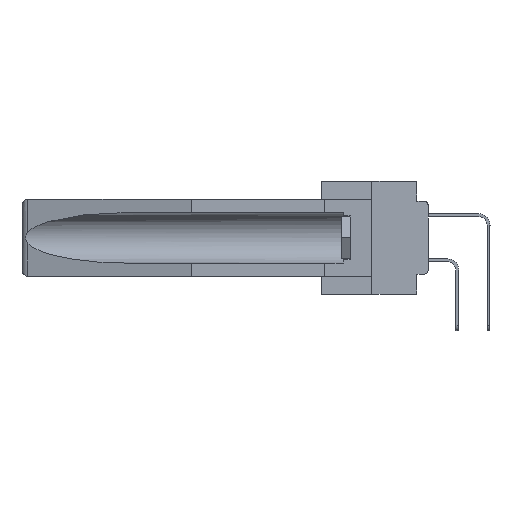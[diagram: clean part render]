
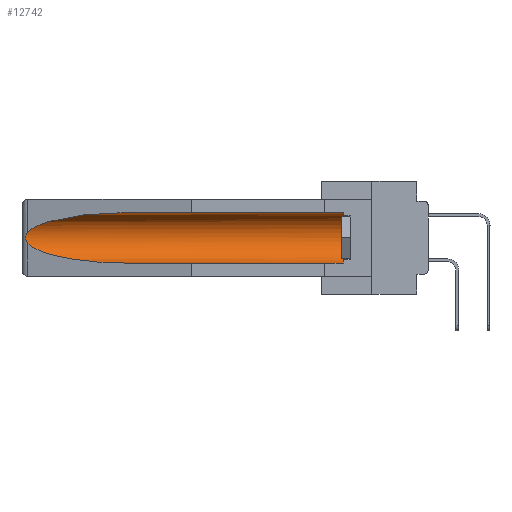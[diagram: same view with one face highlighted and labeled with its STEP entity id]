
A CAD part, left-side view. The second image highlights one B-rep face of the part: STEP entity #12742.
In plain terms, the highlighted cylindrical face has radius 2.857 mm (diameter 5.715 mm), a partial arc.
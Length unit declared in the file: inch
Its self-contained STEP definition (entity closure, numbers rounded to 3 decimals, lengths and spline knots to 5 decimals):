
#198 = CARTESIAN_POINT ( 'NONE',  ( 0.2675, 1.53308, -0.17534 ) ) ;
#292 = EDGE_CURVE ( 'NONE', #12893, #26331, #24643, .T. ) ;
#403 = CARTESIAN_POINT ( 'NONE',  ( 0.26537, 1.52718, -0.14972 ) ) ;
#547 = FACE_OUTER_BOUND ( 'NONE', #8751, .T. ) ;
#893 = CARTESIAN_POINT ( 'NONE',  ( 0.25451, 1.48313, -0.09465 ) ) ;
#2131 = CARTESIAN_POINT ( 'NONE',  ( 0.155, 0.126, -0.284 ) ) ;
#2896 = AXIS2_PLACEMENT_3D ( 'NONE', #5522, #5727, #15255 ) ;
#4227 = CARTESIAN_POINT ( 'NONE',  ( 0.155, 1.07973, -0.059 ) ) ;
#5254 = CARTESIAN_POINT ( 'NONE',  ( 0.2675, 1.53308, -0.16763 ) ) ;
#5522 = CARTESIAN_POINT ( 'NONE',  ( 0.155, -0.30754, -0.1715 ) ) ;
#5727 = DIRECTION ( 'NONE',  ( 0., 1., 0. ) ) ;
#5830 = DIRECTION ( 'NONE',  ( 0., -1., 0. ) ) ;
#6938 = CARTESIAN_POINT ( 'NONE',  ( 0.25451, 1.48313, -0.24835 ) ) ;
#7372 = CARTESIAN_POINT ( 'NONE',  ( 0.26597, 1.52961, -0.15275 ) ) ;
#7940 = AXIS2_PLACEMENT_3D ( 'NONE', #17822, #5830, #15642 ) ;
#8128 = CARTESIAN_POINT ( 'NONE',  ( 0.155, 1.07973, -0.284 ) ) ;
#8637 = DIRECTION ( 'NONE',  ( 0., 1., 0. ) ) ;
#8751 = EDGE_LOOP ( 'NONE', ( #20984, #21102, #9882, #10970, #22609, #20809 ) ) ;
#9882 = ORIENTED_EDGE ( 'NONE', *, *, #29986, .T. ) ;
#9934 = CARTESIAN_POINT ( 'NONE',  ( 0.26537, 1.52718, -0.14972 ) ) ;
#10054 = CARTESIAN_POINT ( 'NONE',  ( 0.26597, 1.5296, -0.19026 ) ) ;
#10134 = LINE ( 'NONE', #17518, #10869 ) ;
#10869 = VECTOR ( 'NONE', #15435, 39.37008 ) ;
#10970 = ORIENTED_EDGE ( 'NONE', *, *, #15511, .F. ) ;
#11609 = VERTEX_POINT ( 'NONE', #4227 ) ;
#12742 = ADVANCED_FACE ( 'NONE', ( #547 ), #20523, .F. ) ;
#12893 = VERTEX_POINT ( 'NONE', #24625 ) ;
#12903 = VERTEX_POINT ( 'NONE', #8128 ) ;
#13728 = VECTOR ( 'NONE', #8637, 39.37008 ) ;
#13769 = CARTESIAN_POINT ( 'NONE',  ( 0.155, 1.07973, -0.284 ) ) ;
#14300 = EDGE_CURVE ( 'NONE', #28640, #11609, #10134, .T. ) ;
#14486 = CARTESIAN_POINT ( 'NONE',  ( 0.21114, 1.30732, -0.059 ) ) ;
#14787 = CARTESIAN_POINT ( 'NONE',  ( 0.26654, 1.53092, -0.15636 ) ) ;
#15255 = DIRECTION ( 'NONE',  ( 0., 0., 1. ) ) ;
#15435 = DIRECTION ( 'NONE',  ( 0., 1., 0. ) ) ;
#15511 = EDGE_CURVE ( 'NONE', #18412, #12903, #24785, .T. ) ;
#15642 = DIRECTION ( 'NONE',  ( 0., 0., 1. ) ) ;
#16315 =( BOUNDED_CURVE ( )  B_SPLINE_CURVE ( 3, ( #19111, #14486, #893, #9934 ),
 .UNSPECIFIED., .F., .F. ) 
 B_SPLINE_CURVE_WITH_KNOTS ( ( 4, 4 ),
 ( 4.71239, 6.08839 ),
 .UNSPECIFIED. ) 
 CURVE ( )  GEOMETRIC_REPRESENTATION_ITEM ( )  RATIONAL_B_SPLINE_CURVE ( ( 1., 0.848, 0.848, 1. ) ) 
 REPRESENTATION_ITEM ( '' )  );
#17518 = CARTESIAN_POINT ( 'NONE',  ( 0.155, -0.30754, -0.059 ) ) ;
#17822 = CARTESIAN_POINT ( 'NONE',  ( 0.155, 0.126, -0.1715 ) ) ;
#18412 = VERTEX_POINT ( 'NONE', #2131 ) ;
#19111 = CARTESIAN_POINT ( 'NONE',  ( 0.155, 1.07973, -0.059 ) ) ;
#20368 = EDGE_CURVE ( 'NONE', #11609, #12893, #16315, .T. ) ;
#20485 =( BOUNDED_CURVE ( )  B_SPLINE_CURVE ( 3, ( #28231, #6938, #28038, #13769 ),
 .UNSPECIFIED., .F., .F. ) 
 B_SPLINE_CURVE_WITH_KNOTS ( ( 4, 4 ),
 ( 0.1948, 1.5708 ),
 .UNSPECIFIED. ) 
 CURVE ( )  GEOMETRIC_REPRESENTATION_ITEM ( )  RATIONAL_B_SPLINE_CURVE ( ( 1., 0.848, 0.848, 1. ) ) 
 REPRESENTATION_ITEM ( '' )  );
#20523 = CYLINDRICAL_SURFACE ( 'NONE', #2896, 0.1125 ) ;
#20611 = CARTESIAN_POINT ( 'NONE',  ( 0.155, -0.30754, -0.284 ) ) ;
#20809 = ORIENTED_EDGE ( 'NONE', *, *, #14300, .T. ) ;
#20984 = ORIENTED_EDGE ( 'NONE', *, *, #20368, .T. ) ;
#21102 = ORIENTED_EDGE ( 'NONE', *, *, #292, .T. ) ;
#21806 = CARTESIAN_POINT ( 'NONE',  ( 0.26655, 1.53094, -0.18657 ) ) ;
#22609 = ORIENTED_EDGE ( 'NONE', *, *, #24699, .T. ) ;
#22824 = CARTESIAN_POINT ( 'NONE',  ( 0.155, 0.126, -0.059 ) ) ;
#24625 = CARTESIAN_POINT ( 'NONE',  ( 0.26537, 1.52718, -0.14972 ) ) ;
#24643 = B_SPLINE_CURVE_WITH_KNOTS ( 'NONE', 3,
 ( #403, #7372, #14787, #28446, #5254, #198, #28648, #21806, #10054, #28747 ),
 .UNSPECIFIED., .F., .F.,
 ( 4, 2, 2, 2, 4 ),
 ( 0., 0.00029, 0.00058, 0.00087, 0.00117 ),
 .UNSPECIFIED. ) ;
#24699 = EDGE_CURVE ( 'NONE', #18412, #28640, #30049, .T. ) ;
#24785 = LINE ( 'NONE', #20611, #13728 ) ;
#26331 = VERTEX_POINT ( 'NONE', #27518 ) ;
#27518 = CARTESIAN_POINT ( 'NONE',  ( 0.26537, 1.52718, -0.19328 ) ) ;
#28038 = CARTESIAN_POINT ( 'NONE',  ( 0.21114, 1.30732, -0.284 ) ) ;
#28231 = CARTESIAN_POINT ( 'NONE',  ( 0.26537, 1.52718, -0.19328 ) ) ;
#28446 = CARTESIAN_POINT ( 'NONE',  ( 0.2673, 1.5327, -0.16383 ) ) ;
#28640 = VERTEX_POINT ( 'NONE', #22824 ) ;
#28648 = CARTESIAN_POINT ( 'NONE',  ( 0.2673, 1.53269, -0.17917 ) ) ;
#28747 = CARTESIAN_POINT ( 'NONE',  ( 0.26537, 1.52718, -0.19328 ) ) ;
#29986 = EDGE_CURVE ( 'NONE', #26331, #12903, #20485, .T. ) ;
#30049 = CIRCLE ( 'NONE', #7940, 0.1125 ) ;
